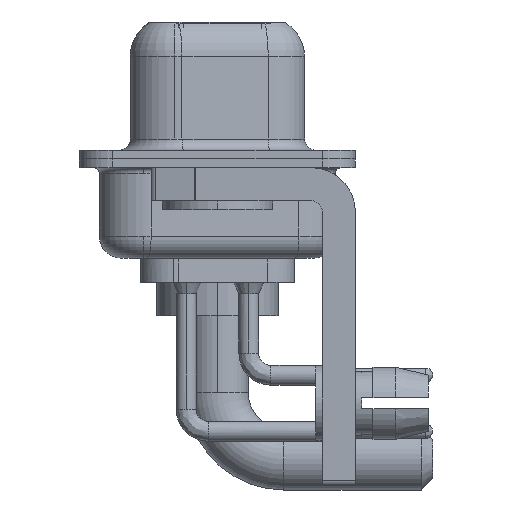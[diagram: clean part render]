
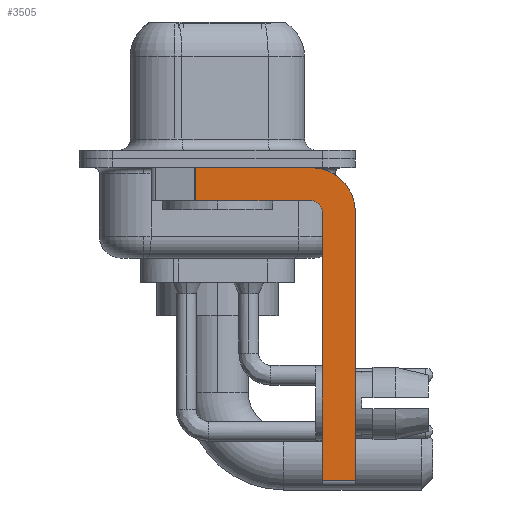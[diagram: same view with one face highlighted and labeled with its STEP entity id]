
A CAD part, left-side view. The second image highlights one B-rep face of the part: STEP entity #3505.
In plain terms, the highlighted planar face has unit normal (-1, 0, 0).
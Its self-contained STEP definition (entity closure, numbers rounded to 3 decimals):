
#924 = DIRECTION ( 'NONE',  ( 0., -1., 0. ) ) ;
#1017 = DIRECTION ( 'NONE',  ( 0., 0., -1. ) ) ;
#1082 = DIRECTION ( 'NONE',  ( -1., 0., 0. ) ) ;
#1305 = VERTEX_POINT ( 'NONE', #9010 ) ;
#1329 = CARTESIAN_POINT ( 'NONE',  ( -2.9, -4.75, -14.55 ) ) ;
#1432 = CARTESIAN_POINT ( 'NONE',  ( -2.9, -4.25, -14.55 ) ) ;
#1583 = CARTESIAN_POINT ( 'NONE',  ( -2.9, -4.25, -1.9 ) ) ;
#1726 = DIRECTION ( 'NONE',  ( 0., -1., 0. ) ) ;
#1973 = FACE_OUTER_BOUND ( 'NONE', #8324, .T. ) ;
#2062 = ORIENTED_EDGE ( 'NONE', *, *, #5917, .F. ) ;
#2398 = ORIENTED_EDGE ( 'NONE', *, *, #8315, .F. ) ;
#2873 = LINE ( 'NONE', #6155, #2932 ) ;
#2932 = VECTOR ( 'NONE', #12600, 1000. ) ;
#2978 = VERTEX_POINT ( 'NONE', #19704 ) ;
#3300 = VERTEX_POINT ( 'NONE', #9511 ) ;
#3505 = ADVANCED_FACE ( 'NONE', ( #1973 ), #8437, .F. ) ;
#3556 = EDGE_CURVE ( 'NONE', #10947, #5139, #18571, .T. ) ;
#3673 = DIRECTION ( 'NONE',  ( 1., 0., 0. ) ) ;
#4015 = CARTESIAN_POINT ( 'NONE',  ( -2.9, -6.25, -2.4 ) ) ;
#4508 = CARTESIAN_POINT ( 'NONE',  ( -2.9, -4.25, -0.4 ) ) ;
#4790 = EDGE_CURVE ( 'NONE', #10477, #15177, #2873, .T. ) ;
#5139 = VERTEX_POINT ( 'NONE', #4015 ) ;
#5477 = AXIS2_PLACEMENT_3D ( 'NONE', #10392, #1082, #15420 ) ;
#5917 = EDGE_CURVE ( 'NONE', #5139, #1305, #14836, .T. ) ;
#6155 = CARTESIAN_POINT ( 'NONE',  ( -2.9, 0.978, -1.9 ) ) ;
#6829 = DIRECTION ( 'NONE',  ( 0., 0., -1. ) ) ;
#7467 = DIRECTION ( 'NONE',  ( 0., 0., -1. ) ) ;
#8315 = EDGE_CURVE ( 'NONE', #10985, #3300, #19656, .T. ) ;
#8324 = EDGE_LOOP ( 'NONE', ( #15857, #14049, #18491, #15028, #2398, #14007, #2062, #12758 ) ) ;
#8437 = PLANE ( 'NONE',  #20590 ) ;
#8976 = LINE ( 'NONE', #16844, #15578 ) ;
#9010 = CARTESIAN_POINT ( 'NONE',  ( -2.9, -6.25, -14.55 ) ) ;
#9511 = CARTESIAN_POINT ( 'NONE',  ( -2.9, -4.75, -2.4 ) ) ;
#10392 = CARTESIAN_POINT ( 'NONE',  ( -2.9, -4.25, -2.4 ) ) ;
#10477 = VERTEX_POINT ( 'NONE', #11399 ) ;
#10757 = VECTOR ( 'NONE', #11796, 1000. ) ;
#10802 = CARTESIAN_POINT ( 'NONE',  ( -2.9, 0.978, -1.9 ) ) ;
#10947 = VERTEX_POINT ( 'NONE', #4508 ) ;
#10971 = LINE ( 'NONE', #1432, #19767 ) ;
#10985 = VERTEX_POINT ( 'NONE', #1329 ) ;
#11399 = CARTESIAN_POINT ( 'NONE',  ( -2.9, 0.978, -0.4 ) ) ;
#11796 = DIRECTION ( 'NONE',  ( 0., 0., 1. ) ) ;
#12032 = CARTESIAN_POINT ( 'NONE',  ( -2.9, -4.25, -2.4 ) ) ;
#12600 = DIRECTION ( 'NONE',  ( 0., 0., -1. ) ) ;
#12758 = ORIENTED_EDGE ( 'NONE', *, *, #3556, .F. ) ;
#13298 = EDGE_CURVE ( 'NONE', #2978, #15177, #20772, .T. ) ;
#13697 = DIRECTION ( 'NONE',  ( 1., 0., 0. ) ) ;
#13878 = VECTOR ( 'NONE', #6829, 1000. ) ;
#14007 = ORIENTED_EDGE ( 'NONE', *, *, #14195, .T. ) ;
#14049 = ORIENTED_EDGE ( 'NONE', *, *, #4790, .T. ) ;
#14195 = EDGE_CURVE ( 'NONE', #10985, #1305, #10971, .T. ) ;
#14476 = DIRECTION ( 'NONE',  ( 0., 1., 0. ) ) ;
#14701 = VECTOR ( 'NONE', #14476, 1000. ) ;
#14836 = LINE ( 'NONE', #19668, #13878 ) ;
#14851 = CARTESIAN_POINT ( 'NONE',  ( -2.9, -4.25, -2.4 ) ) ;
#15028 = ORIENTED_EDGE ( 'NONE', *, *, #20240, .F. ) ;
#15121 = CARTESIAN_POINT ( 'NONE',  ( -2.9, -4.75, -14.8 ) ) ;
#15177 = VERTEX_POINT ( 'NONE', #10802 ) ;
#15420 = DIRECTION ( 'NONE',  ( 0., 0., 1. ) ) ;
#15578 = VECTOR ( 'NONE', #924, 1000. ) ;
#15857 = ORIENTED_EDGE ( 'NONE', *, *, #20649, .F. ) ;
#15894 = CIRCLE ( 'NONE', #5477, 0.5 ) ;
#16240 = AXIS2_PLACEMENT_3D ( 'NONE', #12032, #13697, #7467 ) ;
#16844 = CARTESIAN_POINT ( 'NONE',  ( -2.9, 3., -0.4 ) ) ;
#18491 = ORIENTED_EDGE ( 'NONE', *, *, #13298, .F. ) ;
#18571 = CIRCLE ( 'NONE', #16240, 2. ) ;
#19656 = LINE ( 'NONE', #15121, #10757 ) ;
#19668 = CARTESIAN_POINT ( 'NONE',  ( -2.9, -6.25, -2.4 ) ) ;
#19704 = CARTESIAN_POINT ( 'NONE',  ( -2.9, -4.25, -1.9 ) ) ;
#19767 = VECTOR ( 'NONE', #1726, 1000. ) ;
#20240 = EDGE_CURVE ( 'NONE', #3300, #2978, #15894, .T. ) ;
#20590 = AXIS2_PLACEMENT_3D ( 'NONE', #14851, #3673, #1017 ) ;
#20649 = EDGE_CURVE ( 'NONE', #10477, #10947, #8976, .T. ) ;
#20772 = LINE ( 'NONE', #1583, #14701 ) ;
